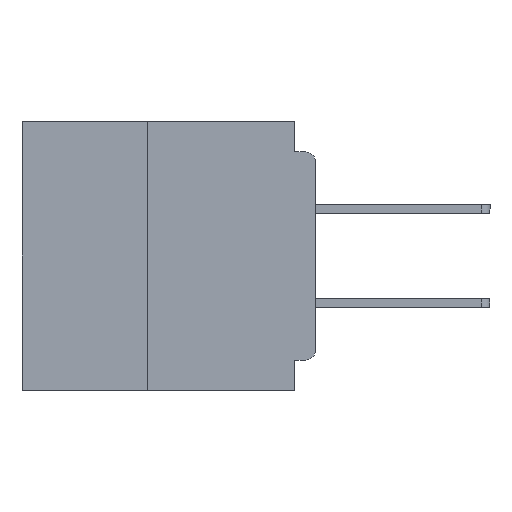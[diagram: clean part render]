
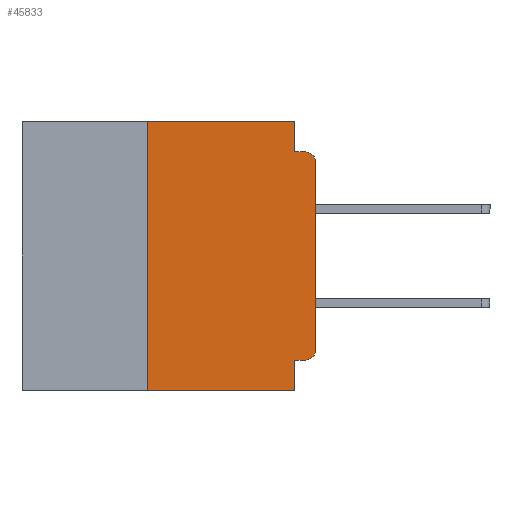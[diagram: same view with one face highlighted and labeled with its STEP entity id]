
A CAD part, left-side view. The second image highlights one B-rep face of the part: STEP entity #45833.
In plain terms, the highlighted planar face has unit normal (-1, 0, 0).
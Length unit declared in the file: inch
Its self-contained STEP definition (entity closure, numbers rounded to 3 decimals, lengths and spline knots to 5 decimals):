
#25 = CARTESIAN_POINT ( 'NONE',  ( 0., 0., -0.06 ) ) ;
#221 = VERTEX_POINT ( 'NONE', #58509 ) ;
#390 = VECTOR ( 'NONE', #53954, 39.37008 ) ;
#877 = CARTESIAN_POINT ( 'NONE',  ( 0., 0.031, 0. ) ) ;
#1046 = AXIS2_PLACEMENT_3D ( 'NONE', #15104, #33736, #24533 ) ;
#1798 = CARTESIAN_POINT ( 'NONE',  ( 0., 0.25, 0. ) ) ;
#2137 = EDGE_CURVE ( 'NONE', #40164, #40289, #48979, .T. ) ;
#2570 = CARTESIAN_POINT ( 'NONE',  ( 0., 0.015, -0.34 ) ) ;
#2997 = EDGE_CURVE ( 'NONE', #59302, #40289, #56844, .T. ) ;
#3087 = VERTEX_POINT ( 'NONE', #27711 ) ;
#3233 = EDGE_CURVE ( 'NONE', #221, #59302, #7921, .T. ) ;
#3529 = ORIENTED_EDGE ( 'NONE', *, *, #44423, .F. ) ;
#4528 = CARTESIAN_POINT ( 'NONE',  ( 0., 0., 0. ) ) ;
#4863 = EDGE_CURVE ( 'NONE', #3087, #31420, #13577, .T. ) ;
#5406 = FACE_OUTER_BOUND ( 'NONE', #55098, .T. ) ;
#7368 = DIRECTION ( 'NONE',  ( 0., 0., -1. ) ) ;
#7613 = CARTESIAN_POINT ( 'NONE',  ( 0., 0.031, 0. ) ) ;
#7921 = LINE ( 'NONE', #24181, #54668 ) ;
#9166 = VECTOR ( 'NONE', #52204, 39.37008 ) ;
#9677 = ORIENTED_EDGE ( 'NONE', *, *, #14285, .T. ) ;
#10549 = CARTESIAN_POINT ( 'NONE',  ( 0., 0., -0.045 ) ) ;
#10557 = ORIENTED_EDGE ( 'NONE', *, *, #46360, .T. ) ;
#12205 = VERTEX_POINT ( 'NONE', #1798 ) ;
#13258 = VERTEX_POINT ( 'NONE', #25 ) ;
#13359 = CARTESIAN_POINT ( 'NONE',  ( 0., 0.015, -0.045 ) ) ;
#13386 = CARTESIAN_POINT ( 'NONE',  ( 0., 0., -0.34 ) ) ;
#13577 = LINE ( 'NONE', #10549, #36942 ) ;
#13845 = VERTEX_POINT ( 'NONE', #13386 ) ;
#14285 = EDGE_CURVE ( 'NONE', #221, #13845, #29363, .T. ) ;
#14763 = DIRECTION ( 'NONE',  ( 0., 1., 0. ) ) ;
#15104 = CARTESIAN_POINT ( 'NONE',  ( 0., 0.437, 0. ) ) ;
#15621 = LINE ( 'NONE', #4528, #51393 ) ;
#16910 = ORIENTED_EDGE ( 'NONE', *, *, #3233, .F. ) ;
#17041 = AXIS2_PLACEMENT_3D ( 'NONE', #2570, #35396, #7368 ) ;
#18875 = EDGE_CURVE ( 'NONE', #34025, #3087, #46760, .T. ) ;
#19839 = PLANE ( 'NONE',  #1046 ) ;
#21992 = VECTOR ( 'NONE', #56909, 39.37008 ) ;
#23462 = DIRECTION ( 'NONE',  ( 0., 0., 1. ) ) ;
#24181 = CARTESIAN_POINT ( 'NONE',  ( 0., 0., -0.355 ) ) ;
#24484 = CARTESIAN_POINT ( 'NONE',  ( 0., 0.015, -0.06 ) ) ;
#24533 = DIRECTION ( 'NONE',  ( 0., 0., -1. ) ) ;
#26080 = CARTESIAN_POINT ( 'NONE',  ( 0., 0.25, -0.4 ) ) ;
#26130 = ORIENTED_EDGE ( 'NONE', *, *, #54671, .T. ) ;
#26952 = LINE ( 'NONE', #26080, #390 ) ;
#27711 = CARTESIAN_POINT ( 'NONE',  ( 0., 0.031, -0.045 ) ) ;
#29197 = DIRECTION ( 'NONE',  ( 0., 0., -1. ) ) ;
#29363 = CIRCLE ( 'NONE', #17041, 0.015 ) ;
#30640 = DIRECTION ( 'NONE',  ( 0., -1., 0. ) ) ;
#31420 = VERTEX_POINT ( 'NONE', #13359 ) ;
#31678 = CARTESIAN_POINT ( 'NONE',  ( 0., 0.031, -0.355 ) ) ;
#32151 = VECTOR ( 'NONE', #41145, 39.37008 ) ;
#32615 = LINE ( 'NONE', #47696, #9166 ) ;
#33719 = VECTOR ( 'NONE', #30640, 39.37008 ) ;
#33736 = DIRECTION ( 'NONE',  ( 1., 0., 0. ) ) ;
#34025 = VERTEX_POINT ( 'NONE', #7613 ) ;
#35316 = CARTESIAN_POINT ( 'NONE',  ( 0., 0.437, -0.4 ) ) ;
#35396 = DIRECTION ( 'NONE',  ( -1., 0., 0. ) ) ;
#36581 = CARTESIAN_POINT ( 'NONE',  ( 0., 0.031, -0.4 ) ) ;
#36942 = VECTOR ( 'NONE', #47859, 39.37008 ) ;
#39784 = CIRCLE ( 'NONE', #40762, 0.015 ) ;
#39812 = ORIENTED_EDGE ( 'NONE', *, *, #50512, .F. ) ;
#40164 = VERTEX_POINT ( 'NONE', #58997 ) ;
#40289 = VERTEX_POINT ( 'NONE', #36581 ) ;
#40762 = AXIS2_PLACEMENT_3D ( 'NONE', #24484, #57038, #29197 ) ;
#41145 = DIRECTION ( 'NONE',  ( 0., 0., -1. ) ) ;
#42685 = ORIENTED_EDGE ( 'NONE', *, *, #2997, .F. ) ;
#42833 = ORIENTED_EDGE ( 'NONE', *, *, #4863, .F. ) ;
#44423 = EDGE_CURVE ( 'NONE', #40164, #12205, #26952, .T. ) ;
#45833 = ADVANCED_FACE ( 'NONE', ( #5406 ), #19839, .F. ) ;
#46360 = EDGE_CURVE ( 'NONE', #13258, #31420, #39784, .T. ) ;
#46760 = LINE ( 'NONE', #877, #21992 ) ;
#47696 = CARTESIAN_POINT ( 'NONE',  ( 0., 0.437, 0. ) ) ;
#47859 = DIRECTION ( 'NONE',  ( 0., -1., 0. ) ) ;
#48979 = LINE ( 'NONE', #35316, #33719 ) ;
#50512 = EDGE_CURVE ( 'NONE', #12205, #34025, #32615, .T. ) ;
#51393 = VECTOR ( 'NONE', #23462, 39.37008 ) ;
#52204 = DIRECTION ( 'NONE',  ( 0., -1., 0. ) ) ;
#53954 = DIRECTION ( 'NONE',  ( 0., 0., 1. ) ) ;
#54668 = VECTOR ( 'NONE', #14763, 39.37008 ) ;
#54671 = EDGE_CURVE ( 'NONE', #13845, #13258, #15621, .T. ) ;
#55098 = EDGE_LOOP ( 'NONE', ( #26130, #10557, #42833, #60642, #39812, #3529, #59073, #42685, #16910, #9677 ) ) ;
#56844 = LINE ( 'NONE', #59844, #32151 ) ;
#56909 = DIRECTION ( 'NONE',  ( 0., 0., -1. ) ) ;
#57038 = DIRECTION ( 'NONE',  ( -1., 0., 0. ) ) ;
#58509 = CARTESIAN_POINT ( 'NONE',  ( 0., 0.015, -0.355 ) ) ;
#58997 = CARTESIAN_POINT ( 'NONE',  ( 0., 0.25, -0.4 ) ) ;
#59073 = ORIENTED_EDGE ( 'NONE', *, *, #2137, .T. ) ;
#59302 = VERTEX_POINT ( 'NONE', #31678 ) ;
#59844 = CARTESIAN_POINT ( 'NONE',  ( 0., 0.031, -0.4 ) ) ;
#60642 = ORIENTED_EDGE ( 'NONE', *, *, #18875, .F. ) ;
